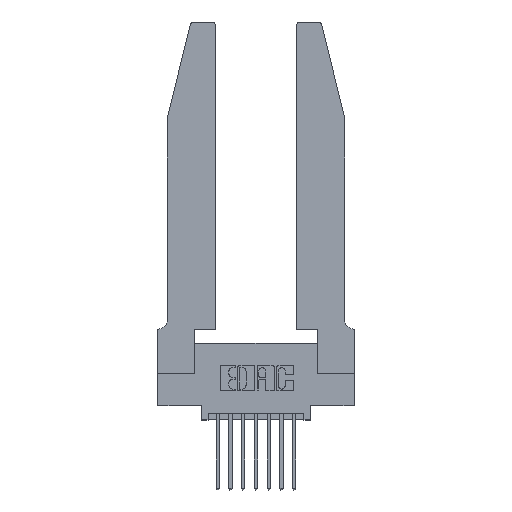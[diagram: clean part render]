
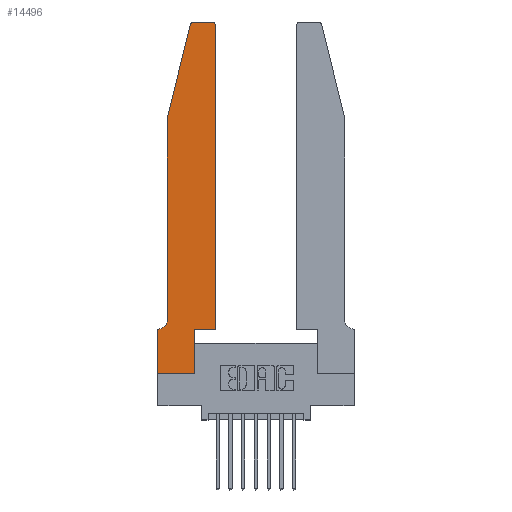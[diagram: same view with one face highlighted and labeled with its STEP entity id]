
A CAD part, top view. The second image highlights one B-rep face of the part: STEP entity #14496.
In plain terms, the highlighted planar face has unit normal (0, 0, 1).
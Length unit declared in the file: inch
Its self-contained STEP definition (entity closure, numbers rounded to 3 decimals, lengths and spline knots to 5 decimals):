
#2 = VERTEX_POINT ( 'NONE', #258 ) ;
#37 = DIRECTION ( 'NONE',  ( 0., 0., 1. ) ) ;
#93 = AXIS2_PLACEMENT_3D ( 'NONE', #9984, #2951, #13619 ) ;
#258 = CARTESIAN_POINT ( 'NONE',  ( 0.284, 2.75, 0.37 ) ) ;
#311 = CARTESIAN_POINT ( 'NONE',  ( 0.0755, 2., 0.37 ) ) ;
#313 = AXIS2_PLACEMENT_3D ( 'NONE', #13508, #11187, #8799 ) ;
#788 = VERTEX_POINT ( 'NONE', #5137 ) ;
#971 = ORIENTED_EDGE ( 'NONE', *, *, #11996, .T. ) ;
#1067 = VECTOR ( 'NONE', #10456, 39.37008 ) ;
#1204 = VERTEX_POINT ( 'NONE', #7652 ) ;
#1271 = CARTESIAN_POINT ( 'NONE',  ( 0.0755, 2., 0.37 ) ) ;
#2161 = VERTEX_POINT ( 'NONE', #5328 ) ;
#2204 = CARTESIAN_POINT ( 'NONE',  ( 0., 0.35, 0.37 ) ) ;
#2501 = ORIENTED_EDGE ( 'NONE', *, *, #2986, .T. ) ;
#2513 = EDGE_CURVE ( 'NONE', #5589, #2, #15021, .T. ) ;
#2844 = DIRECTION ( 'NONE',  ( -0.239, -0.971, 0. ) ) ;
#2951 = DIRECTION ( 'NONE',  ( 0., 0., 1. ) ) ;
#2986 = EDGE_CURVE ( 'NONE', #10366, #14685, #3859, .T. ) ;
#3095 = CARTESIAN_POINT ( 'NONE',  ( 0.25487, 2.72718, 0.37 ) ) ;
#3223 = ORIENTED_EDGE ( 'NONE', *, *, #5354, .T. ) ;
#3226 = CARTESIAN_POINT ( 'NONE',  ( 0.2605, 2.75, 0.37 ) ) ;
#3250 = CARTESIAN_POINT ( 'NONE',  ( 0., 0., 0.37 ) ) ;
#3335 = VECTOR ( 'NONE', #12736, 39.37008 ) ;
#3526 = CARTESIAN_POINT ( 'NONE',  ( 0.0755, 0.35, 0.37 ) ) ;
#3747 = DIRECTION ( 'NONE',  ( 0., -1., 0. ) ) ;
#3859 = LINE ( 'NONE', #12590, #3335 ) ;
#3895 = ORIENTED_EDGE ( 'NONE', *, *, #10649, .T. ) ;
#3957 = CARTESIAN_POINT ( 'NONE',  ( 0.0755, 2., 0.37 ) ) ;
#4127 = EDGE_CURVE ( 'NONE', #14685, #5589, #14412, .T. ) ;
#4150 = ORIENTED_EDGE ( 'NONE', *, *, #9296, .T. ) ;
#4190 = FACE_OUTER_BOUND ( 'NONE', #7064, .T. ) ;
#4228 = ORIENTED_EDGE ( 'NONE', *, *, #15053, .T. ) ;
#4931 = VECTOR ( 'NONE', #3747, 39.37008 ) ;
#5137 = CARTESIAN_POINT ( 'NONE',  ( 0., 0., 0.37 ) ) ;
#5328 = CARTESIAN_POINT ( 'NONE',  ( 0., 0.35, 0.37 ) ) ;
#5337 = VECTOR ( 'NONE', #6531, 39.37008 ) ;
#5354 = EDGE_CURVE ( 'NONE', #1204, #2161, #9834, .T. ) ;
#5535 = EDGE_CURVE ( 'NONE', #10841, #10366, #11099, .T. ) ;
#5589 = VERTEX_POINT ( 'NONE', #11132 ) ;
#5759 = CARTESIAN_POINT ( 'NONE',  ( 0.4205, 2.72, 0.37 ) ) ;
#5911 = VECTOR ( 'NONE', #13530, 39.37008 ) ;
#6209 = ORIENTED_EDGE ( 'NONE', *, *, #14579, .T. ) ;
#6426 = ORIENTED_EDGE ( 'NONE', *, *, #5535, .T. ) ;
#6475 = CARTESIAN_POINT ( 'NONE',  ( 0.0755, 0.42, 0.37 ) ) ;
#6531 = DIRECTION ( 'NONE',  ( 0., -1., 0. ) ) ;
#6626 = CARTESIAN_POINT ( 'NONE',  ( 0.4505, 0.35, 0.37 ) ) ;
#6730 = VECTOR ( 'NONE', #8376, 39.37008 ) ;
#6988 = CARTESIAN_POINT ( 'NONE',  ( 0.4505, 0.35, 0.37 ) ) ;
#7064 = EDGE_LOOP ( 'NONE', ( #11540, #13405, #971, #6209, #3895, #3223, #12921, #4150, #4228, #6426, #2501, #11984 ) ) ;
#7524 = VERTEX_POINT ( 'NONE', #11391 ) ;
#7638 = VECTOR ( 'NONE', #13713, 39.37008 ) ;
#7652 = CARTESIAN_POINT ( 'NONE',  ( 0.0055, 0.35, 0.37 ) ) ;
#7829 = LINE ( 'NONE', #9018, #7638 ) ;
#7891 = DIRECTION ( 'NONE',  ( 1., 0., 0. ) ) ;
#7939 = DIRECTION ( 'NONE',  ( 0., 0., 1. ) ) ;
#8300 = EDGE_CURVE ( 'NONE', #2, #13653, #11403, .T. ) ;
#8376 = DIRECTION ( 'NONE',  ( -1., 0., 0. ) ) ;
#8387 = LINE ( 'NONE', #1271, #4931 ) ;
#8663 = AXIS2_PLACEMENT_3D ( 'NONE', #5759, #7939, #7891 ) ;
#8799 = DIRECTION ( 'NONE',  ( -1., 0., 0. ) ) ;
#9018 = CARTESIAN_POINT ( 'NONE',  ( 0.2865, 0.35, 0.37 ) ) ;
#9296 = EDGE_CURVE ( 'NONE', #788, #7524, #13395, .T. ) ;
#9834 = LINE ( 'NONE', #3526, #6730 ) ;
#9984 = CARTESIAN_POINT ( 'NONE',  ( 0.284, 2.72, 0.37 ) ) ;
#10279 = EDGE_CURVE ( 'NONE', #2161, #788, #10426, .T. ) ;
#10366 = VERTEX_POINT ( 'NONE', #6626 ) ;
#10386 = VECTOR ( 'NONE', #2844, 39.37008 ) ;
#10426 = LINE ( 'NONE', #3250, #5337 ) ;
#10456 = DIRECTION ( 'NONE',  ( 1., 0., 0. ) ) ;
#10649 = EDGE_CURVE ( 'NONE', #13014, #1204, #10969, .T. ) ;
#10841 = VERTEX_POINT ( 'NONE', #13604 ) ;
#10969 = CIRCLE ( 'NONE', #313, 0.07 ) ;
#11099 = LINE ( 'NONE', #6988, #1067 ) ;
#11132 = CARTESIAN_POINT ( 'NONE',  ( 0.4205, 2.75, 0.37 ) ) ;
#11187 = DIRECTION ( 'NONE',  ( 0., 0., -1. ) ) ;
#11391 = CARTESIAN_POINT ( 'NONE',  ( 0.2865, 0., 0.37 ) ) ;
#11403 = CIRCLE ( 'NONE', #93, 0.03 ) ;
#11528 = DIRECTION ( 'NONE',  ( 1., 0., 0. ) ) ;
#11540 = ORIENTED_EDGE ( 'NONE', *, *, #2513, .T. ) ;
#11978 = CARTESIAN_POINT ( 'NONE',  ( 0.4505, 2.72, 0.37 ) ) ;
#11984 = ORIENTED_EDGE ( 'NONE', *, *, #4127, .T. ) ;
#11996 = EDGE_CURVE ( 'NONE', #13653, #13461, #13507, .T. ) ;
#12254 = AXIS2_PLACEMENT_3D ( 'NONE', #2204, #37, #11528 ) ;
#12590 = CARTESIAN_POINT ( 'NONE',  ( 0.4505, 0.35, 0.37 ) ) ;
#12736 = DIRECTION ( 'NONE',  ( 0., 1., 0. ) ) ;
#12921 = ORIENTED_EDGE ( 'NONE', *, *, #10279, .T. ) ;
#13014 = VERTEX_POINT ( 'NONE', #6475 ) ;
#13395 = LINE ( 'NONE', #13421, #5911 ) ;
#13405 = ORIENTED_EDGE ( 'NONE', *, *, #8300, .T. ) ;
#13421 = CARTESIAN_POINT ( 'NONE',  ( 0., 0., 0.37 ) ) ;
#13461 = VERTEX_POINT ( 'NONE', #311 ) ;
#13507 = LINE ( 'NONE', #3957, #10386 ) ;
#13508 = CARTESIAN_POINT ( 'NONE',  ( 0.0055, 0.42, 0.37 ) ) ;
#13530 = DIRECTION ( 'NONE',  ( 1., 0., 0. ) ) ;
#13584 = VECTOR ( 'NONE', #14513, 39.37008 ) ;
#13604 = CARTESIAN_POINT ( 'NONE',  ( 0.2865, 0.35, 0.37 ) ) ;
#13619 = DIRECTION ( 'NONE',  ( 1., 0., 0. ) ) ;
#13653 = VERTEX_POINT ( 'NONE', #3095 ) ;
#13713 = DIRECTION ( 'NONE',  ( 0., 1., 0. ) ) ;
#13972 = PLANE ( 'NONE',  #12254 ) ;
#14412 = CIRCLE ( 'NONE', #8663, 0.03 ) ;
#14496 = ADVANCED_FACE ( 'NONE', ( #4190 ), #13972, .T. ) ;
#14513 = DIRECTION ( 'NONE',  ( -1., 0., 0. ) ) ;
#14579 = EDGE_CURVE ( 'NONE', #13461, #13014, #8387, .T. ) ;
#14685 = VERTEX_POINT ( 'NONE', #11978 ) ;
#15021 = LINE ( 'NONE', #3226, #13584 ) ;
#15053 = EDGE_CURVE ( 'NONE', #7524, #10841, #7829, .T. ) ;
